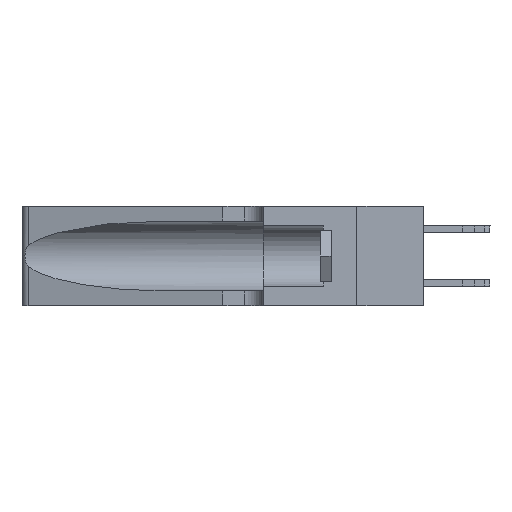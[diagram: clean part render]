
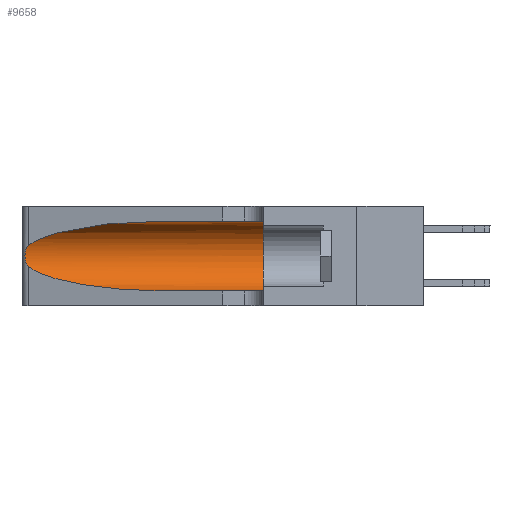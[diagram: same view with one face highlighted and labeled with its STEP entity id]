
A CAD part, left-side view. The second image highlights one B-rep face of the part: STEP entity #9658.
In plain terms, the highlighted cylindrical face has radius 3.308 mm (diameter 6.617 mm), a partial arc.
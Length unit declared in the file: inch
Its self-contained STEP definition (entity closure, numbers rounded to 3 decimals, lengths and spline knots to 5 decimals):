
#467 = CARTESIAN_POINT ( 'NONE',  ( 0.25789, 1.23486, 0.15765 ) ) ;
#625 = EDGE_CURVE ( 'NONE', #25041, #8401, #2441, .T. ) ;
#1372 = CARTESIAN_POINT ( 'NONE',  ( 0.18966, 0.96281, 0.31525 ) ) ;
#2441 = B_SPLINE_CURVE_WITH_KNOTS ( 'NONE', 3,
 ( #17053, #12334, #26613, #12545, #28987, #2941, #28683, #29091, #14579, #2739, #467, #14890, #5198, #26504 ),
 .UNSPECIFIED., .F., .F.,
 ( 4, 2, 2, 2, 2, 2, 4 ),
 ( 0., 0.00027, 0.00053, 0.00107, 0.0016, 0.00187, 0.00214 ),
 .UNSPECIFIED. ) ;
#2739 = CARTESIAN_POINT ( 'NONE',  ( 0.25856, 1.23593, 0.16098 ) ) ;
#2829 = CYLINDRICAL_SURFACE ( 'NONE', #27306, 0.13025 ) ;
#2941 = CARTESIAN_POINT ( 'NONE',  ( 0.26018, 1.23835, 0.19895 ) ) ;
#5122 = EDGE_CURVE ( 'NONE', #23694, #16549, #22287, .T. ) ;
#5198 = CARTESIAN_POINT ( 'NONE',  ( 0.25555, 1.22993, 0.14849 ) ) ;
#5432 = DIRECTION ( 'NONE',  ( 0., 0., -1. ) ) ;
#5675 = ORIENTED_EDGE ( 'NONE', *, *, #18039, .F. ) ;
#6768 = VECTOR ( 'NONE', #14121, 39.37008 ) ;
#7235 = CARTESIAN_POINT ( 'NONE',  ( 0.25487, 1.22718, 0.14631 ) ) ;
#7553 = CARTESIAN_POINT ( 'NONE',  ( 0.1305, 0.72297, 0.05475 ) ) ;
#8212 = ORIENTED_EDGE ( 'NONE', *, *, #625, .T. ) ;
#8401 = VERTEX_POINT ( 'NONE', #10936 ) ;
#8559 = ORIENTED_EDGE ( 'NONE', *, *, #22289, .T. ) ;
#8969 = EDGE_LOOP ( 'NONE', ( #18089, #8212, #8559, #25959, #30438, #5675 ) ) ;
#9658 = ADVANCED_FACE ( 'NONE', ( #10946 ), #2829, .F. ) ;
#9941 = CARTESIAN_POINT ( 'NONE',  ( 0.2373, 1.15595, 0.08982 ) ) ;
#10936 = CARTESIAN_POINT ( 'NONE',  ( 0.25487, 1.22718, 0.14631 ) ) ;
#10946 = FACE_OUTER_BOUND ( 'NONE', #8969, .T. ) ;
#11015 = CARTESIAN_POINT ( 'NONE',  ( 0.25487, 1.22718, 0.22369 ) ) ;
#12334 = CARTESIAN_POINT ( 'NONE',  ( 0.25555, 1.22994, 0.2215 ) ) ;
#12515 = CARTESIAN_POINT ( 'NONE',  ( 0.1305, 0.35, 0.05475 ) ) ;
#12545 = CARTESIAN_POINT ( 'NONE',  ( 0.25787, 1.23484, 0.2124 ) ) ;
#13863 = CARTESIAN_POINT ( 'NONE',  ( 0.1305, 0.35, 0.31525 ) ) ;
#14121 = DIRECTION ( 'NONE',  ( 0., -1., 0. ) ) ;
#14360 = DIRECTION ( 'NONE',  ( 0., 1., 0. ) ) ;
#14495 = DIRECTION ( 'NONE',  ( 0., -1., 0. ) ) ;
#14579 = CARTESIAN_POINT ( 'NONE',  ( 0.26017, 1.23833, 0.17102 ) ) ;
#14889 = CARTESIAN_POINT ( 'NONE',  ( 0.1305, 1.61858, 0.31525 ) ) ;
#14890 = CARTESIAN_POINT ( 'NONE',  ( 0.25639, 1.23186, 0.15144 ) ) ;
#16191 = CARTESIAN_POINT ( 'NONE',  ( 0.1305, 0.72297, 0.31525 ) ) ;
#16265 = CARTESIAN_POINT ( 'NONE',  ( 0.1305, 1.61858, 0.05475 ) ) ;
#16549 = VERTEX_POINT ( 'NONE', #12515 ) ;
#16962 = CARTESIAN_POINT ( 'NONE',  ( 0.1305, 1.61858, 0.185 ) ) ;
#17053 = CARTESIAN_POINT ( 'NONE',  ( 0.25487, 1.22718, 0.22369 ) ) ;
#17866 = CARTESIAN_POINT ( 'NONE',  ( 0.25487, 1.22718, 0.22369 ) ) ;
#18039 = EDGE_CURVE ( 'NONE', #20613, #18401, #29625, .T. ) ;
#18089 = ORIENTED_EDGE ( 'NONE', *, *, #20564, .T. ) ;
#18401 = VERTEX_POINT ( 'NONE', #13863 ) ;
#19507 = DIRECTION ( 'NONE',  ( 0., -1., 0. ) ) ;
#20131 = CARTESIAN_POINT ( 'NONE',  ( 0.1305, 0.72297, 0.31525 ) ) ;
#20327 = CARTESIAN_POINT ( 'NONE',  ( 0.2373, 1.15595, 0.28018 ) ) ;
#20564 = EDGE_CURVE ( 'NONE', #20613, #25041, #22638, .T. ) ;
#20613 = VERTEX_POINT ( 'NONE', #16191 ) ;
#21340 = CARTESIAN_POINT ( 'NONE',  ( 0.18966, 0.96281, 0.05475 ) ) ;
#22287 = LINE ( 'NONE', #16265, #6768 ) ;
#22289 = EDGE_CURVE ( 'NONE', #8401, #23694, #27553, .T. ) ;
#22638 =( BOUNDED_CURVE ( )  B_SPLINE_CURVE ( 3, ( #20131, #1372, #20327, #17866 ),
 .UNSPECIFIED., .F., .F. ) 
 B_SPLINE_CURVE_WITH_KNOTS ( ( 4, 4 ),
 ( 1.5708, 2.84003 ),
 .UNSPECIFIED. ) 
 CURVE ( )  GEOMETRIC_REPRESENTATION_ITEM ( )  RATIONAL_B_SPLINE_CURVE ( ( 1., 0.87, 0.87, 1. ) ) 
 REPRESENTATION_ITEM ( '' )  );
#23694 = VERTEX_POINT ( 'NONE', #27134 ) ;
#23902 = DIRECTION ( 'NONE',  ( 0., 0., 1. ) ) ;
#24789 = CARTESIAN_POINT ( 'NONE',  ( 0.1305, 0.35, 0.185 ) ) ;
#25041 = VERTEX_POINT ( 'NONE', #11015 ) ;
#25899 = AXIS2_PLACEMENT_3D ( 'NONE', #24789, #14360, #23902 ) ;
#25959 = ORIENTED_EDGE ( 'NONE', *, *, #5122, .T. ) ;
#26007 = CIRCLE ( 'NONE', #25899, 0.13025 ) ;
#26504 = CARTESIAN_POINT ( 'NONE',  ( 0.25487, 1.22718, 0.14631 ) ) ;
#26613 = CARTESIAN_POINT ( 'NONE',  ( 0.25639, 1.23184, 0.21858 ) ) ;
#27134 = CARTESIAN_POINT ( 'NONE',  ( 0.1305, 0.72297, 0.05475 ) ) ;
#27306 = AXIS2_PLACEMENT_3D ( 'NONE', #16962, #14495, #5432 ) ;
#27394 = VECTOR ( 'NONE', #19507, 39.37008 ) ;
#27553 =( BOUNDED_CURVE ( )  B_SPLINE_CURVE ( 3, ( #7235, #9941, #21340, #7553 ),
 .UNSPECIFIED., .F., .F. ) 
 B_SPLINE_CURVE_WITH_KNOTS ( ( 4, 4 ),
 ( 3.44316, 4.71239 ),
 .UNSPECIFIED. ) 
 CURVE ( )  GEOMETRIC_REPRESENTATION_ITEM ( )  RATIONAL_B_SPLINE_CURVE ( ( 1., 0.87, 0.87, 1. ) ) 
 REPRESENTATION_ITEM ( '' )  );
#28683 = CARTESIAN_POINT ( 'NONE',  ( 0.26075, 1.23896, 0.19203 ) ) ;
#28987 = CARTESIAN_POINT ( 'NONE',  ( 0.25854, 1.2359, 0.20912 ) ) ;
#29091 = CARTESIAN_POINT ( 'NONE',  ( 0.26075, 1.23896, 0.178 ) ) ;
#29625 = LINE ( 'NONE', #14889, #27394 ) ;
#30397 = EDGE_CURVE ( 'NONE', #18401, #16549, #26007, .T. ) ;
#30438 = ORIENTED_EDGE ( 'NONE', *, *, #30397, .F. ) ;
